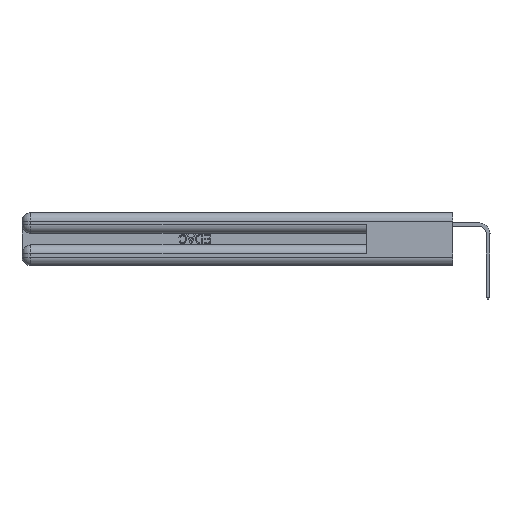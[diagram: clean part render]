
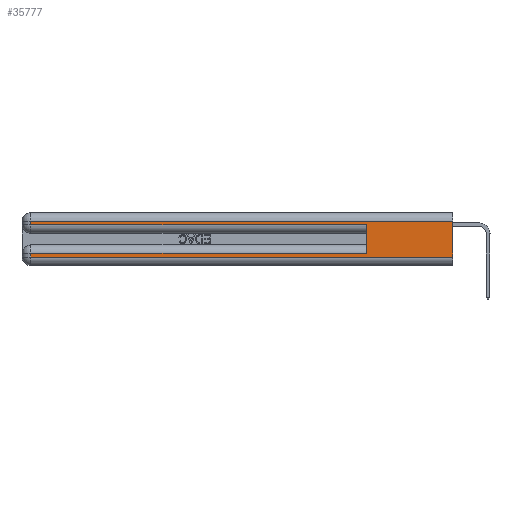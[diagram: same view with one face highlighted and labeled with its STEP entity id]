
A CAD part, left-side view. The second image highlights one B-rep face of the part: STEP entity #35777.
In plain terms, the highlighted planar face has unit normal (-1, 0, 0).
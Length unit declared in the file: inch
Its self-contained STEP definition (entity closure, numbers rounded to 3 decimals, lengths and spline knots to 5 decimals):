
#3516 = CARTESIAN_POINT ( 'NONE',  ( 0., 0., 0.085 ) ) ;
#4047 = VERTEX_POINT ( 'NONE', #32026 ) ;
#4519 = DIRECTION ( 'NONE',  ( 0., 1., 0. ) ) ;
#4602 = CARTESIAN_POINT ( 'NONE',  ( 0., 0., 0.06 ) ) ;
#4683 = EDGE_CURVE ( 'NONE', #18762, #13396, #31668, .T. ) ;
#5546 = DIRECTION ( 'NONE',  ( 0., 0., -1. ) ) ;
#5863 = CARTESIAN_POINT ( 'NONE',  ( 0., 0., 0.06 ) ) ;
#5885 = CARTESIAN_POINT ( 'NONE',  ( 0., 2.94, 0.31 ) ) ;
#6012 = PLANE ( 'NONE',  #31096 ) ;
#6212 = LINE ( 'NONE', #5863, #22238 ) ;
#6299 = EDGE_LOOP ( 'NONE', ( #19449, #28914, #13561, #30930, #10150, #35999, #22113, #37502 ) ) ;
#6925 = LINE ( 'NONE', #12255, #22909 ) ;
#6983 = CARTESIAN_POINT ( 'NONE',  ( 0., 2.94, 0.37 ) ) ;
#7195 = VERTEX_POINT ( 'NONE', #21206 ) ;
#7703 = DIRECTION ( 'NONE',  ( 0., -1., 0. ) ) ;
#8107 = VERTEX_POINT ( 'NONE', #5885 ) ;
#9163 = DIRECTION ( 'NONE',  ( 0., -1., 0. ) ) ;
#9291 = DIRECTION ( 'NONE',  ( 0., 0., -1. ) ) ;
#10150 = ORIENTED_EDGE ( 'NONE', *, *, #4683, .F. ) ;
#10385 = CARTESIAN_POINT ( 'NONE',  ( 0., 2.94, 0.06 ) ) ;
#10641 = LINE ( 'NONE', #3516, #26539 ) ;
#11112 = VERTEX_POINT ( 'NONE', #4602 ) ;
#12255 = CARTESIAN_POINT ( 'NONE',  ( 0., 0., 0.37 ) ) ;
#12326 = LINE ( 'NONE', #6983, #28206 ) ;
#12359 = CARTESIAN_POINT ( 'NONE',  ( 0., 0.6, 0.145 ) ) ;
#13396 = VERTEX_POINT ( 'NONE', #30746 ) ;
#13561 = ORIENTED_EDGE ( 'NONE', *, *, #28238, .T. ) ;
#13798 = LINE ( 'NONE', #14031, #29667 ) ;
#13821 = VECTOR ( 'NONE', #18759, 39.37008 ) ;
#14031 = CARTESIAN_POINT ( 'NONE',  ( 0., 0., 0.285 ) ) ;
#14159 = EDGE_CURVE ( 'NONE', #28251, #11112, #6212, .T. ) ;
#15577 = DIRECTION ( 'NONE',  ( 0., 0., -1. ) ) ;
#17251 = VERTEX_POINT ( 'NONE', #21278 ) ;
#17632 = EDGE_CURVE ( 'NONE', #17251, #13396, #13798, .T. ) ;
#17839 = CARTESIAN_POINT ( 'NONE',  ( 0., 0.6, 0.085 ) ) ;
#18759 = DIRECTION ( 'NONE',  ( 0., 0., 1. ) ) ;
#18762 = VERTEX_POINT ( 'NONE', #17839 ) ;
#19449 = ORIENTED_EDGE ( 'NONE', *, *, #21100, .F. ) ;
#20657 = CARTESIAN_POINT ( 'NONE',  ( 0., 0., 0.31 ) ) ;
#20763 = LINE ( 'NONE', #24853, #29200 ) ;
#21100 = EDGE_CURVE ( 'NONE', #7195, #11112, #6925, .T. ) ;
#21206 = CARTESIAN_POINT ( 'NONE',  ( 0., 0., 0.31 ) ) ;
#21278 = CARTESIAN_POINT ( 'NONE',  ( 0., 2.94, 0.285 ) ) ;
#22113 = ORIENTED_EDGE ( 'NONE', *, *, #24798, .T. ) ;
#22238 = VECTOR ( 'NONE', #9163, 39.37008 ) ;
#22708 = DIRECTION ( 'NONE',  ( 0., 1., 0. ) ) ;
#22909 = VECTOR ( 'NONE', #15577, 39.37008 ) ;
#24565 = FACE_OUTER_BOUND ( 'NONE', #6299, .T. ) ;
#24798 = EDGE_CURVE ( 'NONE', #4047, #28251, #20763, .T. ) ;
#24853 = CARTESIAN_POINT ( 'NONE',  ( 0., 2.94, 0.37 ) ) ;
#26094 = DIRECTION ( 'NONE',  ( 0., 0., -1. ) ) ;
#26539 = VECTOR ( 'NONE', #22708, 39.37008 ) ;
#26917 = EDGE_CURVE ( 'NONE', #18762, #4047, #10641, .T. ) ;
#28206 = VECTOR ( 'NONE', #26094, 39.37008 ) ;
#28238 = EDGE_CURVE ( 'NONE', #8107, #17251, #12326, .T. ) ;
#28251 = VERTEX_POINT ( 'NONE', #10385 ) ;
#28332 = DIRECTION ( 'NONE',  ( 1., 0., 0. ) ) ;
#28914 = ORIENTED_EDGE ( 'NONE', *, *, #36764, .T. ) ;
#29200 = VECTOR ( 'NONE', #5546, 39.37008 ) ;
#29667 = VECTOR ( 'NONE', #7703, 39.37008 ) ;
#30746 = CARTESIAN_POINT ( 'NONE',  ( 0., 0.6, 0.285 ) ) ;
#30912 = LINE ( 'NONE', #20657, #39394 ) ;
#30930 = ORIENTED_EDGE ( 'NONE', *, *, #17632, .T. ) ;
#31096 = AXIS2_PLACEMENT_3D ( 'NONE', #37768, #28332, #9291 ) ;
#31668 = LINE ( 'NONE', #12359, #13821 ) ;
#32026 = CARTESIAN_POINT ( 'NONE',  ( 0., 2.94, 0.085 ) ) ;
#35777 = ADVANCED_FACE ( 'NONE', ( #24565 ), #6012, .F. ) ;
#35999 = ORIENTED_EDGE ( 'NONE', *, *, #26917, .T. ) ;
#36764 = EDGE_CURVE ( 'NONE', #7195, #8107, #30912, .T. ) ;
#37502 = ORIENTED_EDGE ( 'NONE', *, *, #14159, .T. ) ;
#37768 = CARTESIAN_POINT ( 'NONE',  ( 0., 0., 0.37 ) ) ;
#39394 = VECTOR ( 'NONE', #4519, 39.37008 ) ;
